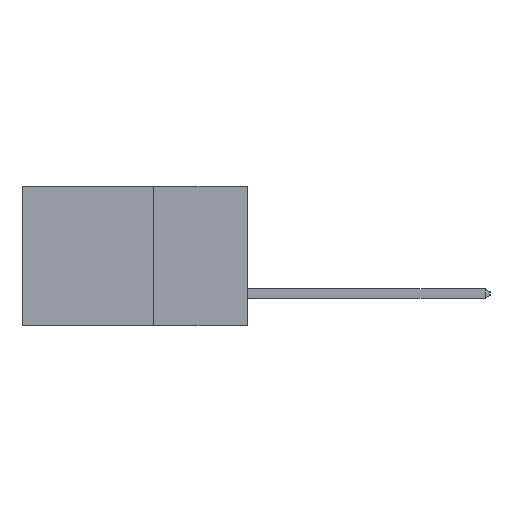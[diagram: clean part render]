
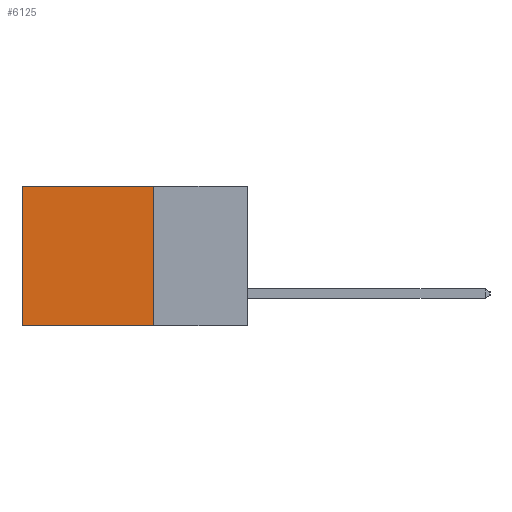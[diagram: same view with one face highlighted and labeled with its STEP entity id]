
A CAD part, left-side view. The second image highlights one B-rep face of the part: STEP entity #6125.
In plain terms, the highlighted planar face has unit normal (-1, 0, 0).
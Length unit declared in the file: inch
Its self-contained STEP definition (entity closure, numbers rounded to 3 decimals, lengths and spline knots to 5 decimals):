
#491 = CARTESIAN_POINT ( 'NONE',  ( 0.2615, 0.25, 0. ) ) ;
#893 = EDGE_LOOP ( 'NONE', ( #5497, #12952, #6868, #15343 ) ) ;
#1331 = LINE ( 'NONE', #7384, #11590 ) ;
#1503 = VERTEX_POINT ( 'NONE', #2727 ) ;
#1605 = VERTEX_POINT ( 'NONE', #491 ) ;
#2727 = CARTESIAN_POINT ( 'NONE',  ( 0.2615, 0.25, -0.37 ) ) ;
#2858 = CARTESIAN_POINT ( 'NONE',  ( 0.2615, 0.6, -0.37 ) ) ;
#3632 = AXIS2_PLACEMENT_3D ( 'NONE', #10951, #5633, #14953 ) ;
#3652 = EDGE_CURVE ( 'NONE', #1605, #14464, #16090, .T. ) ;
#4794 = CARTESIAN_POINT ( 'NONE',  ( 0.2615, 0.25, 0. ) ) ;
#5165 = EDGE_CURVE ( 'NONE', #1503, #10965, #12733, .T. ) ;
#5497 = ORIENTED_EDGE ( 'NONE', *, *, #15887, .T. ) ;
#5633 = DIRECTION ( 'NONE',  ( 1., 0., 0. ) ) ;
#6125 = ADVANCED_FACE ( 'NONE', ( #14576 ), #13632, .F. ) ;
#6391 = DIRECTION ( 'NONE',  ( 0., 1., 0. ) ) ;
#6592 = VECTOR ( 'NONE', #15074, 39.37008 ) ;
#6868 = ORIENTED_EDGE ( 'NONE', *, *, #15991, .F. ) ;
#7088 = CARTESIAN_POINT ( 'NONE',  ( 0.2615, 0.6, -0.37 ) ) ;
#7384 = CARTESIAN_POINT ( 'NONE',  ( 0.2615, 0.25, -0.37 ) ) ;
#8722 = DIRECTION ( 'NONE',  ( 0., 0., -1. ) ) ;
#9237 = VECTOR ( 'NONE', #6391, 39.37008 ) ;
#10150 = LINE ( 'NONE', #7088, #6592 ) ;
#10951 = CARTESIAN_POINT ( 'NONE',  ( 0.2615, 0.25, -0.37 ) ) ;
#10965 = VERTEX_POINT ( 'NONE', #2858 ) ;
#11590 = VECTOR ( 'NONE', #8722, 39.37008 ) ;
#12580 = VECTOR ( 'NONE', #14132, 39.37008 ) ;
#12733 = LINE ( 'NONE', #13031, #9237 ) ;
#12952 = ORIENTED_EDGE ( 'NONE', *, *, #5165, .F. ) ;
#13031 = CARTESIAN_POINT ( 'NONE',  ( 0.2615, 0.25, -0.37 ) ) ;
#13632 = PLANE ( 'NONE',  #3632 ) ;
#14132 = DIRECTION ( 'NONE',  ( 0., 1., 0. ) ) ;
#14438 = CARTESIAN_POINT ( 'NONE',  ( 0.2615, 0.6, 0. ) ) ;
#14464 = VERTEX_POINT ( 'NONE', #14438 ) ;
#14576 = FACE_OUTER_BOUND ( 'NONE', #893, .T. ) ;
#14953 = DIRECTION ( 'NONE',  ( 0., 0., -1. ) ) ;
#15074 = DIRECTION ( 'NONE',  ( 0., 0., -1. ) ) ;
#15343 = ORIENTED_EDGE ( 'NONE', *, *, #3652, .T. ) ;
#15887 = EDGE_CURVE ( 'NONE', #14464, #10965, #10150, .T. ) ;
#15991 = EDGE_CURVE ( 'NONE', #1605, #1503, #1331, .T. ) ;
#16090 = LINE ( 'NONE', #4794, #12580 ) ;
